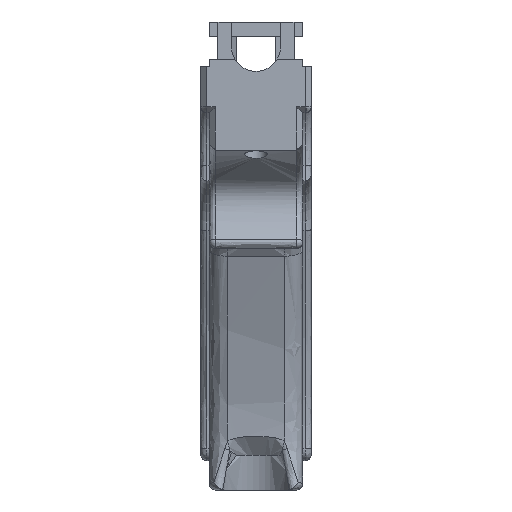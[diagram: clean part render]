
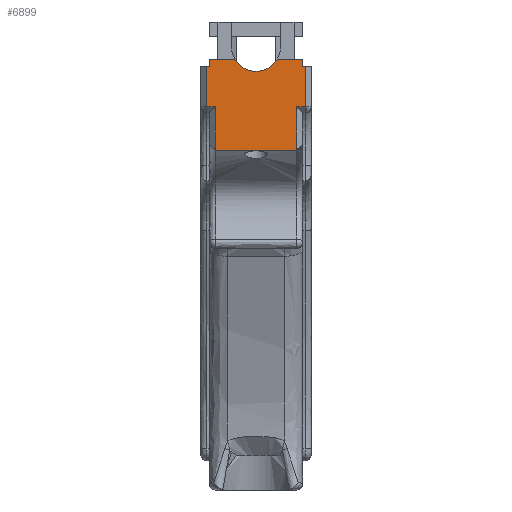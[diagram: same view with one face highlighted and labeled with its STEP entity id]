
A CAD part, front view. The second image highlights one B-rep face of the part: STEP entity #6899.
In plain terms, the highlighted planar face has unit normal (0, -1, 0).
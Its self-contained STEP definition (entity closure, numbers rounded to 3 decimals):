
#553=PLANE('',#7383);
#885=FACE_OUTER_BOUND('',#1275,.T.);
#1275=EDGE_LOOP('',(#6248,#6249,#6250,#6251,#6252,#6253,#6254,#6255,#6256,
#6257,#6258,#6259,#6260,#6261,#6262,#6263));
#1820=LINE('',#13861,#2460);
#1823=LINE('',#13867,#2463);
#1828=LINE('',#13879,#2468);
#1831=LINE('',#13884,#2471);
#1833=LINE('',#13888,#2473);
#1834=LINE('',#13890,#2474);
#1835=LINE('',#13893,#2475);
#1837=LINE('',#13897,#2477);
#1840=LINE('',#13902,#2480);
#1841=LINE('',#13904,#2481);
#1843=LINE('',#13929,#2483);
#1923=LINE('',#14505,#2563);
#1930=LINE('',#14519,#2570);
#1932=LINE('',#14523,#2572);
#1933=LINE('',#14524,#2573);
#2460=VECTOR('',#8615,10.);
#2463=VECTOR('',#8620,10.);
#2468=VECTOR('',#8631,10.);
#2471=VECTOR('',#8636,10.);
#2473=VECTOR('',#8640,10.);
#2474=VECTOR('',#8643,10.);
#2475=VECTOR('',#8646,10.);
#2477=VECTOR('',#8650,10.);
#2480=VECTOR('',#8655,10.);
#2481=VECTOR('',#8658,10.);
#2483=VECTOR('',#8664,10.);
#2563=VECTOR('',#8860,10.);
#2570=VECTOR('',#8871,10.);
#2572=VECTOR('',#8875,10.);
#2573=VECTOR('',#8876,10.);
#2742=CIRCLE('',#7312,4.2);
#3125=VERTEX_POINT('',#12211);
#3320=VERTEX_POINT('',#13858);
#3321=VERTEX_POINT('',#13860);
#3323=VERTEX_POINT('',#13866);
#3325=VERTEX_POINT('',#13872);
#3326=VERTEX_POINT('',#13874);
#3327=VERTEX_POINT('',#13878);
#3328=VERTEX_POINT('',#13882);
#3329=VERTEX_POINT('',#13886);
#3330=VERTEX_POINT('',#13892);
#3331=VERTEX_POINT('',#13896);
#3332=VERTEX_POINT('',#13900);
#3336=VERTEX_POINT('',#13928);
#3405=VERTEX_POINT('',#14504);
#3410=VERTEX_POINT('',#14517);
#3411=VERTEX_POINT('',#14522);
#4238=EDGE_CURVE('',#3321,#3320,#1820,.T.);
#4241=EDGE_CURVE('',#3321,#3323,#1823,.T.);
#4245=EDGE_CURVE('',#3326,#3325,#2742,.T.);
#4247=EDGE_CURVE('',#3326,#3327,#1828,.T.);
#4250=EDGE_CURVE('',#3327,#3328,#1831,.T.);
#4252=EDGE_CURVE('',#3329,#3328,#1833,.T.);
#4253=EDGE_CURVE('',#3329,#3125,#1834,.T.);
#4254=EDGE_CURVE('',#3125,#3330,#1835,.T.);
#4256=EDGE_CURVE('',#3330,#3331,#1837,.T.);
#4259=EDGE_CURVE('',#3331,#3332,#1840,.F.);
#4260=EDGE_CURVE('',#3320,#3332,#1841,.T.);
#4265=EDGE_CURVE('',#3323,#3336,#1843,.T.);
#4379=EDGE_CURVE('',#3405,#3325,#1923,.T.);
#4386=EDGE_CURVE('',#3410,#3405,#1930,.T.);
#4388=EDGE_CURVE('',#3410,#3411,#1932,.T.);
#4389=EDGE_CURVE('',#3336,#3411,#1933,.T.);
#6248=ORIENTED_EDGE('',*,*,#4260,.T.);
#6249=ORIENTED_EDGE('',*,*,#4259,.F.);
#6250=ORIENTED_EDGE('',*,*,#4256,.F.);
#6251=ORIENTED_EDGE('',*,*,#4254,.F.);
#6252=ORIENTED_EDGE('',*,*,#4253,.F.);
#6253=ORIENTED_EDGE('',*,*,#4252,.T.);
#6254=ORIENTED_EDGE('',*,*,#4250,.F.);
#6255=ORIENTED_EDGE('',*,*,#4247,.F.);
#6256=ORIENTED_EDGE('',*,*,#4245,.T.);
#6257=ORIENTED_EDGE('',*,*,#4379,.F.);
#6258=ORIENTED_EDGE('',*,*,#4386,.F.);
#6259=ORIENTED_EDGE('',*,*,#4388,.T.);
#6260=ORIENTED_EDGE('',*,*,#4389,.F.);
#6261=ORIENTED_EDGE('',*,*,#4265,.F.);
#6262=ORIENTED_EDGE('',*,*,#4241,.F.);
#6263=ORIENTED_EDGE('',*,*,#4238,.T.);
#6899=ADVANCED_FACE('',(#885),#553,.T.);
#7312=AXIS2_PLACEMENT_3D('',#13875,#8626,#8627);
#7383=AXIS2_PLACEMENT_3D('',#14521,#8873,#8874);
#8615=DIRECTION('',(0.707,0.,-0.707));
#8620=DIRECTION('',(0.,0.,1.));
#8626=DIRECTION('center_axis',(0.,1.,0.));
#8627=DIRECTION('ref_axis',(1.,0.,0.));
#8631=DIRECTION('',(1.,0.,0.));
#8636=DIRECTION('',(0.,0.,-1.));
#8640=DIRECTION('',(-1.,0.,0.));
#8643=DIRECTION('',(0.,0.,-1.));
#8646=DIRECTION('',(-1.,0.,0.));
#8650=DIRECTION('',(0.,0.,-1.));
#8655=DIRECTION('',(0.707,0.,0.707));
#8658=DIRECTION('',(1.,0.,0.));
#8664=DIRECTION('',(-1.,0.,0.));
#8860=DIRECTION('',(1.,0.,0.));
#8871=DIRECTION('',(0.,0.,1.));
#8873=DIRECTION('center_axis',(0.,-1.,0.));
#8874=DIRECTION('ref_axis',(0.,0.,-1.));
#8875=DIRECTION('',(-1.,0.,0.));
#8876=DIRECTION('',(0.,0.,1.));
#12211=CARTESIAN_POINT('',(16.4,-118.,-4.6));
#13858=CARTESIAN_POINT('',(1.057,-118.,-12.057));
#13860=CARTESIAN_POINT('',(1.,-118.,-12.));
#13861=CARTESIAN_POINT('',(-3.375,-118.,-7.625));
#13866=CARTESIAN_POINT('',(1.,-118.,-4.6));
#13867=CARTESIAN_POINT('',(1.,-118.,-7.95));
#13872=CARTESIAN_POINT('',(4.356,-118.,3.5));
#13874=CARTESIAN_POINT('',(11.544,-118.,3.5));
#13875=CARTESIAN_POINT('Origin',(7.95,-118.,5.673));
#13878=CARTESIAN_POINT('',(15.9,-118.,3.5));
#13879=CARTESIAN_POINT('',(0.,-118.,3.5));
#13882=CARTESIAN_POINT('',(15.9,-118.,2.25));
#13884=CARTESIAN_POINT('',(15.9,-118.,5.1));
#13886=CARTESIAN_POINT('',(16.4,-118.,2.25));
#13888=CARTESIAN_POINT('',(17.4,-118.,2.25));
#13890=CARTESIAN_POINT('',(16.4,-118.,0.413));
#13892=CARTESIAN_POINT('',(14.9,-118.,-4.6));
#13893=CARTESIAN_POINT('',(0.725,-118.,-4.6));
#13896=CARTESIAN_POINT('',(14.9,-118.,-12.));
#13897=CARTESIAN_POINT('',(14.9,-118.,5.1));
#13900=CARTESIAN_POINT('',(14.843,-118.,-12.057));
#13902=CARTESIAN_POINT('',(15.3,-118.,-11.6));
#13904=CARTESIAN_POINT('',(3.974,-118.,-12.057));
#13928=CARTESIAN_POINT('',(-0.5,-118.,-4.6));
#13929=CARTESIAN_POINT('',(0.725,-118.,-4.6));
#14504=CARTESIAN_POINT('',(0.,-118.,3.5));
#14505=CARTESIAN_POINT('',(0.,-118.,3.5));
#14517=CARTESIAN_POINT('',(0.,-118.,2.25));
#14519=CARTESIAN_POINT('',(0.,-118.,-7.95));
#14521=CARTESIAN_POINT('Origin',(0.,-118.,3.5));
#14522=CARTESIAN_POINT('',(-0.5,-118.,2.25));
#14523=CARTESIAN_POINT('',(-1.5,-118.,2.25));
#14524=CARTESIAN_POINT('',(-0.5,-118.,0.413));
